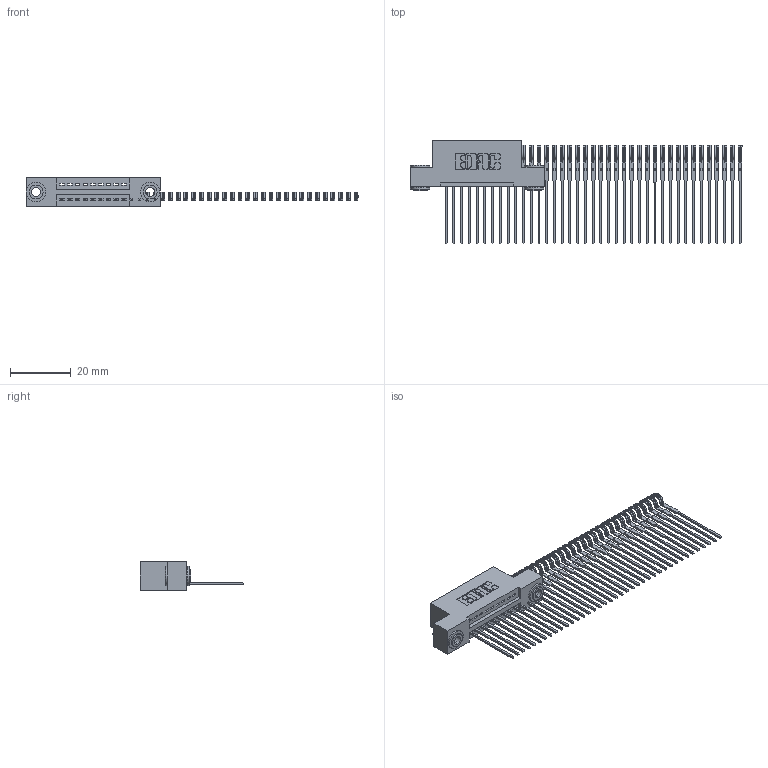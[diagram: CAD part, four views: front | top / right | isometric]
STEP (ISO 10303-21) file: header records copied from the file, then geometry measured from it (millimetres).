
FILE_DESCRIPTION (( 'STEP AP203' ), '1' );
FILE_NAME ('345-039-541-103.STEP', '2018-08-31T23:46:47', ( '' ), ( '' ), 'SwSTEP 2.0', 'SolidWorks 2016', '' );
FILE_SCHEMA (( 'CONFIG_CONTROL_DESIGN' ));
Length unit declared in the file: inch
Products named in the file (4): 345 Part_Flush Mounting Lugs - 0.156 Dia-TH; 345-292-001_345-293-141; 345-250-002_345-250-002-102; 345-039-541-103
Assembly tree (42 placements, depth 2):
  345-039-541-103
    345 Part_Flush Mounting Lugs - 0.156 Dia-TH
    345-292-001_345-293-141  x39
    345-250-002_345-250-002-102  x2
Bounding box: 109.03 x 33.96 x 9.4 mm (x, y, z)
Volume: 4407 mm3; surface area: 8204 mm2
Topology: 42 solids, 42 shells, 1946 faces, 5661 edges, 3718 vertices
Faces by surface type: plane 1230, cylinder 708, cone 8
Entity records: 12844 total; most frequent: CARTESIAN_POINT 2068, ORIENTED_EDGE 1974, DIRECTION 1919, EDGE_CURVE 987, VECTOR 795, LINE 795, VERTEX_POINT 654, AXIS2_PLACEMENT_3D 562
